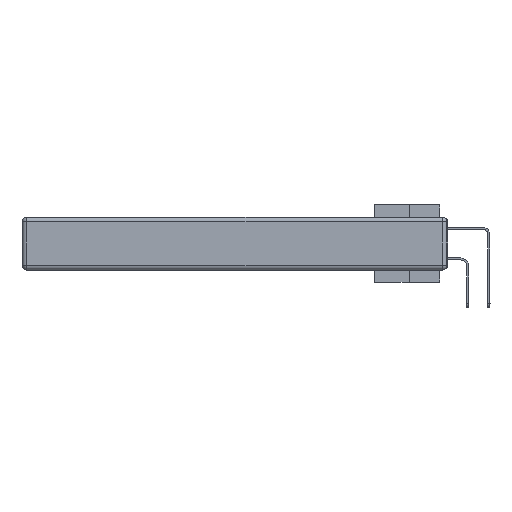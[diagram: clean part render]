
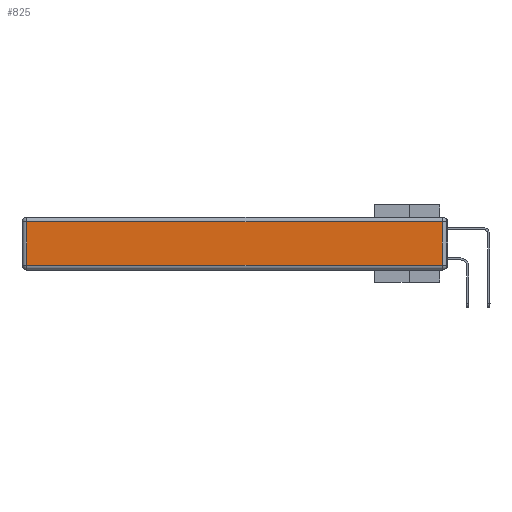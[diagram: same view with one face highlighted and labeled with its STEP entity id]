
A CAD part, left-side view. The second image highlights one B-rep face of the part: STEP entity #825.
In plain terms, the highlighted planar face has unit normal (-1, 0, 0).
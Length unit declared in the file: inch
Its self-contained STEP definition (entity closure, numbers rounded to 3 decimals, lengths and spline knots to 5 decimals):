
#825 = ADVANCED_FACE ( 'NONE', ( #29792 ), #12252, .T. ) ;
#914 = CARTESIAN_POINT ( 'NONE',  ( 0., 2.72, -0.03 ) ) ;
#1225 = VECTOR ( 'NONE', #8833, 39.37008 ) ;
#1585 = EDGE_LOOP ( 'NONE', ( #17284, #8440, #22795, #7221 ) ) ;
#3047 = CARTESIAN_POINT ( 'NONE',  ( 0., 0.03, -0.313 ) ) ;
#3252 = VERTEX_POINT ( 'NONE', #3047 ) ;
#3370 = VERTEX_POINT ( 'NONE', #914 ) ;
#3629 = DIRECTION ( 'NONE',  ( 0., 0., 1. ) ) ;
#3682 = DIRECTION ( 'NONE',  ( 0., 0., 1. ) ) ;
#3848 = CARTESIAN_POINT ( 'NONE',  ( 0., 0.03, -0.343 ) ) ;
#6004 = EDGE_CURVE ( 'NONE', #30054, #3252, #10476, .T. ) ;
#6203 = EDGE_CURVE ( 'NONE', #24967, #3370, #31288, .T. ) ;
#7221 = ORIENTED_EDGE ( 'NONE', *, *, #31069, .T. ) ;
#8037 = VECTOR ( 'NONE', #18532, 39.37008 ) ;
#8440 = ORIENTED_EDGE ( 'NONE', *, *, #25826, .T. ) ;
#8833 = DIRECTION ( 'NONE',  ( 0., 1., 0. ) ) ;
#9487 = VECTOR ( 'NONE', #3682, 39.37008 ) ;
#10476 = LINE ( 'NONE', #16054, #8037 ) ;
#12252 = PLANE ( 'NONE',  #28278 ) ;
#13599 = CARTESIAN_POINT ( 'NONE',  ( 0., 0.03, -0.03 ) ) ;
#14696 = CARTESIAN_POINT ( 'NONE',  ( 0., 2.72, -0.343 ) ) ;
#16054 = CARTESIAN_POINT ( 'NONE',  ( 0., 0., -0.313 ) ) ;
#16130 = VECTOR ( 'NONE', #27791, 39.37008 ) ;
#17284 = ORIENTED_EDGE ( 'NONE', *, *, #6004, .T. ) ;
#18532 = DIRECTION ( 'NONE',  ( 0., -1., 0. ) ) ;
#18629 = LINE ( 'NONE', #3848, #9487 ) ;
#21379 = CARTESIAN_POINT ( 'NONE',  ( 0., 2.72, -0.313 ) ) ;
#22247 = CARTESIAN_POINT ( 'NONE',  ( 0., 0., -0.343 ) ) ;
#22795 = ORIENTED_EDGE ( 'NONE', *, *, #6203, .T. ) ;
#24967 = VERTEX_POINT ( 'NONE', #13599 ) ;
#25826 = EDGE_CURVE ( 'NONE', #3252, #24967, #18629, .T. ) ;
#26070 = DIRECTION ( 'NONE',  ( -1., 0., 0. ) ) ;
#27465 = LINE ( 'NONE', #14696, #16130 ) ;
#27791 = DIRECTION ( 'NONE',  ( 0., 0., -1. ) ) ;
#28278 = AXIS2_PLACEMENT_3D ( 'NONE', #22247, #26070, #3629 ) ;
#29792 = FACE_OUTER_BOUND ( 'NONE', #1585, .T. ) ;
#30054 = VERTEX_POINT ( 'NONE', #21379 ) ;
#31069 = EDGE_CURVE ( 'NONE', #3370, #30054, #27465, .T. ) ;
#31288 = LINE ( 'NONE', #31606, #1225 ) ;
#31606 = CARTESIAN_POINT ( 'NONE',  ( 0., 2.75, -0.03 ) ) ;
